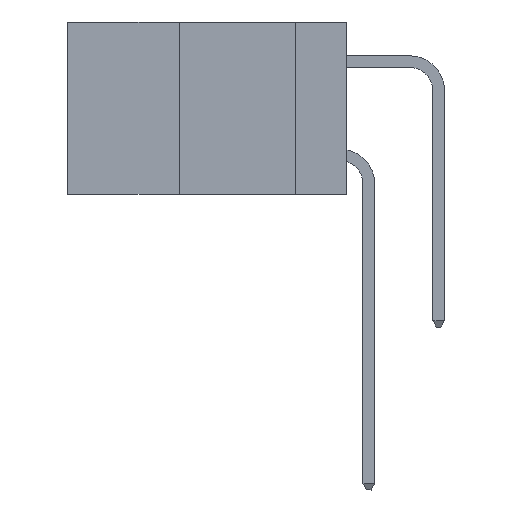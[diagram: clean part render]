
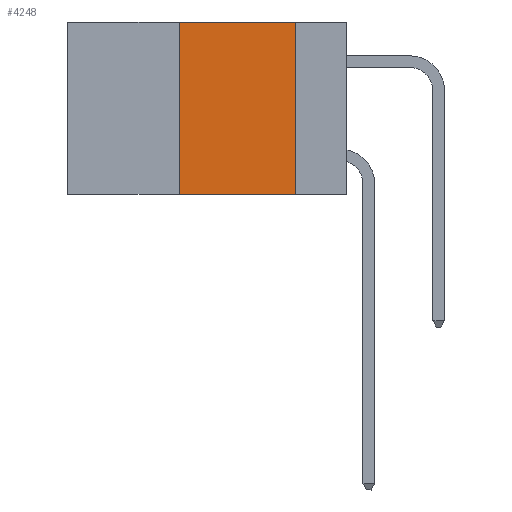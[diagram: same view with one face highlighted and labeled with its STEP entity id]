
A CAD part, left-side view. The second image highlights one B-rep face of the part: STEP entity #4248.
In plain terms, the highlighted planar face has unit normal (-1, 0, 0).
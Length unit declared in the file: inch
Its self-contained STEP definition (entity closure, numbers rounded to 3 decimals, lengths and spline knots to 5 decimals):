
#790 = VECTOR ( 'NONE', #10843, 39.37008 ) ;
#802 = LINE ( 'NONE', #7432, #1698 ) ;
#1229 = FACE_OUTER_BOUND ( 'NONE', #12410, .T. ) ;
#1365 = VERTEX_POINT ( 'NONE', #5167 ) ;
#1432 = DIRECTION ( 'NONE',  ( 0., -1., 0. ) ) ;
#1698 = VECTOR ( 'NONE', #19017, 39.37008 ) ;
#2292 = CARTESIAN_POINT ( 'NONE',  ( 0., 0.11, 0. ) ) ;
#2666 = CARTESIAN_POINT ( 'NONE',  ( 0., 0.6, 0. ) ) ;
#2973 = CARTESIAN_POINT ( 'NONE',  ( 0., 0.6, -0.37 ) ) ;
#3363 = LINE ( 'NONE', #8470, #14774 ) ;
#3616 = VECTOR ( 'NONE', #1432, 39.37008 ) ;
#4248 = ADVANCED_FACE ( 'NONE', ( #1229 ), #21079, .F. ) ;
#4395 = EDGE_CURVE ( 'NONE', #1365, #14931, #19655, .T. ) ;
#5167 = CARTESIAN_POINT ( 'NONE',  ( 0., 0.36, -0.37 ) ) ;
#7339 = LINE ( 'NONE', #17722, #790 ) ;
#7432 = CARTESIAN_POINT ( 'NONE',  ( 0., 0.6, 0. ) ) ;
#7506 = EDGE_CURVE ( 'NONE', #1365, #18629, #3363, .T. ) ;
#7545 = DIRECTION ( 'NONE',  ( 0., 0., -1. ) ) ;
#8438 = VERTEX_POINT ( 'NONE', #2292 ) ;
#8470 = CARTESIAN_POINT ( 'NONE',  ( 0., 0.36, 0. ) ) ;
#8631 = ORIENTED_EDGE ( 'NONE', *, *, #9935, .F. ) ;
#9159 = AXIS2_PLACEMENT_3D ( 'NONE', #2666, #12576, #7545 ) ;
#9935 = EDGE_CURVE ( 'NONE', #18629, #8438, #802, .T. ) ;
#10005 = DIRECTION ( 'NONE',  ( 0., 0., 1. ) ) ;
#10843 = DIRECTION ( 'NONE',  ( 0., 0., -1. ) ) ;
#12410 = EDGE_LOOP ( 'NONE', ( #14159, #8631, #16048, #13246 ) ) ;
#12576 = DIRECTION ( 'NONE',  ( 1., 0., 0. ) ) ;
#13246 = ORIENTED_EDGE ( 'NONE', *, *, #4395, .T. ) ;
#14159 = ORIENTED_EDGE ( 'NONE', *, *, #19429, .F. ) ;
#14176 = CARTESIAN_POINT ( 'NONE',  ( 0., 0.36, 0. ) ) ;
#14774 = VECTOR ( 'NONE', #10005, 39.37008 ) ;
#14931 = VERTEX_POINT ( 'NONE', #21182 ) ;
#16048 = ORIENTED_EDGE ( 'NONE', *, *, #7506, .F. ) ;
#17722 = CARTESIAN_POINT ( 'NONE',  ( 0., 0.11, 0. ) ) ;
#18629 = VERTEX_POINT ( 'NONE', #14176 ) ;
#19017 = DIRECTION ( 'NONE',  ( 0., -1., 0. ) ) ;
#19429 = EDGE_CURVE ( 'NONE', #8438, #14931, #7339, .T. ) ;
#19655 = LINE ( 'NONE', #2973, #3616 ) ;
#21079 = PLANE ( 'NONE',  #9159 ) ;
#21182 = CARTESIAN_POINT ( 'NONE',  ( 0., 0.11, -0.37 ) ) ;
